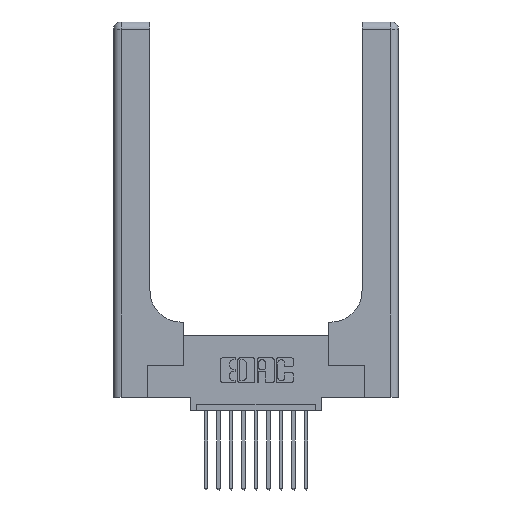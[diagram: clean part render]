
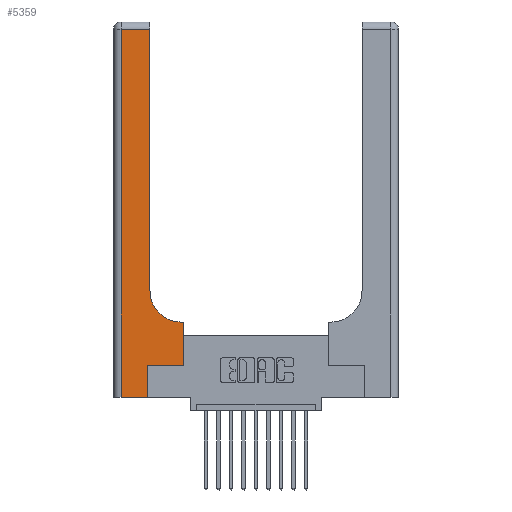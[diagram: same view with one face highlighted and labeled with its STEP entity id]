
A CAD part, top view. The second image highlights one B-rep face of the part: STEP entity #5359.
In plain terms, the highlighted planar face has unit normal (0, 0, 1).
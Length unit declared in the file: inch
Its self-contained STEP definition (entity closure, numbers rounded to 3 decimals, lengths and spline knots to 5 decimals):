
#34 = CARTESIAN_POINT ( 'NONE',  ( 0.2915, 0.6, 0.37 ) ) ;
#67 = EDGE_CURVE ( 'NONE', #10072, #5061, #8543, .T. ) ;
#112 = CARTESIAN_POINT ( 'NONE',  ( 0.5585, 0.25, 0.37 ) ) ;
#182 = ORIENTED_EDGE ( 'NONE', *, *, #4690, .T. ) ;
#774 = VERTEX_POINT ( 'NONE', #4327 ) ;
#806 = CARTESIAN_POINT ( 'NONE',  ( 0.2915, 3., 0.37 ) ) ;
#816 = CARTESIAN_POINT ( 'NONE',  ( 0.5415, 0.85, 0.37 ) ) ;
#1166 = CARTESIAN_POINT ( 'NONE',  ( 0.06, 2.94, 0.37 ) ) ;
#1419 = CARTESIAN_POINT ( 'NONE',  ( 0.269, 0.25, 0.37 ) ) ;
#1625 = EDGE_LOOP ( 'NONE', ( #16168, #10044, #14314, #6061, #182, #9993, #2555, #4718, #5748 ) ) ;
#1907 = AXIS2_PLACEMENT_3D ( 'NONE', #7122, #12544, #11205 ) ;
#2036 = DIRECTION ( 'NONE',  ( 1., 0., 0. ) ) ;
#2192 = VECTOR ( 'NONE', #16117, 39.37008 ) ;
#2379 = LINE ( 'NONE', #13437, #4820 ) ;
#2392 = LINE ( 'NONE', #16055, #7996 ) ;
#2555 = ORIENTED_EDGE ( 'NONE', *, *, #5330, .T. ) ;
#2706 = LINE ( 'NONE', #4996, #12505 ) ;
#2727 = DIRECTION ( 'NONE',  ( -1., 0., 0. ) ) ;
#3348 = DIRECTION ( 'NONE',  ( 0., 1., 0. ) ) ;
#3488 = DIRECTION ( 'NONE',  ( 1., 0., 0. ) ) ;
#3876 = CARTESIAN_POINT ( 'NONE',  ( 0.06, 3., 0.37 ) ) ;
#4117 = CARTESIAN_POINT ( 'NONE',  ( 0.269, 0., 0.37 ) ) ;
#4118 = CARTESIAN_POINT ( 'NONE',  ( 0.5415, 0.6, 0.37 ) ) ;
#4327 = CARTESIAN_POINT ( 'NONE',  ( 0.5585, 0.6, 0.37 ) ) ;
#4550 = AXIS2_PLACEMENT_3D ( 'NONE', #816, #9803, #3488 ) ;
#4690 = EDGE_CURVE ( 'NONE', #7204, #10072, #6435, .T. ) ;
#4718 = ORIENTED_EDGE ( 'NONE', *, *, #11504, .T. ) ;
#4820 = VECTOR ( 'NONE', #2036, 39.37008 ) ;
#4972 = LINE ( 'NONE', #3876, #14729 ) ;
#4996 = CARTESIAN_POINT ( 'NONE',  ( 0., 2.94, 0.37 ) ) ;
#5061 = VERTEX_POINT ( 'NONE', #112 ) ;
#5330 = EDGE_CURVE ( 'NONE', #5061, #774, #2392, .T. ) ;
#5359 = ADVANCED_FACE ( 'NONE', ( #16391 ), #13480, .F. ) ;
#5748 = ORIENTED_EDGE ( 'NONE', *, *, #10424, .T. ) ;
#6056 = DIRECTION ( 'NONE',  ( 1., 0., 0. ) ) ;
#6061 = ORIENTED_EDGE ( 'NONE', *, *, #14273, .T. ) ;
#6435 = LINE ( 'NONE', #4117, #12404 ) ;
#6474 = DIRECTION ( 'NONE',  ( -1., 0., 0. ) ) ;
#6517 = CIRCLE ( 'NONE', #4550, 0.25 ) ;
#6578 = CARTESIAN_POINT ( 'NONE',  ( 0.269, 0.25, 0.37 ) ) ;
#7122 = CARTESIAN_POINT ( 'NONE',  ( 0., 3., 0.37 ) ) ;
#7204 = VERTEX_POINT ( 'NONE', #14443 ) ;
#7996 = VECTOR ( 'NONE', #3348, 39.37008 ) ;
#8191 = LINE ( 'NONE', #806, #2192 ) ;
#8480 = VERTEX_POINT ( 'NONE', #12617 ) ;
#8543 = LINE ( 'NONE', #6578, #14733 ) ;
#8684 = CARTESIAN_POINT ( 'NONE',  ( 0.06, 0., 0.37 ) ) ;
#9544 = VERTEX_POINT ( 'NONE', #12246 ) ;
#9803 = DIRECTION ( 'NONE',  ( 0., 0., -1. ) ) ;
#9993 = ORIENTED_EDGE ( 'NONE', *, *, #67, .T. ) ;
#10044 = ORIENTED_EDGE ( 'NONE', *, *, #11347, .T. ) ;
#10072 = VERTEX_POINT ( 'NONE', #1419 ) ;
#10278 = DIRECTION ( 'NONE',  ( 0., -1., 0. ) ) ;
#10424 = EDGE_CURVE ( 'NONE', #15781, #8480, #6517, .T. ) ;
#11205 = DIRECTION ( 'NONE',  ( -1., 0., 0. ) ) ;
#11347 = EDGE_CURVE ( 'NONE', #9544, #14542, #2706, .T. ) ;
#11461 = VERTEX_POINT ( 'NONE', #8684 ) ;
#11504 = EDGE_CURVE ( 'NONE', #774, #15781, #13903, .T. ) ;
#12246 = CARTESIAN_POINT ( 'NONE',  ( 0.2915, 2.94, 0.37 ) ) ;
#12404 = VECTOR ( 'NONE', #13872, 39.37008 ) ;
#12505 = VECTOR ( 'NONE', #2727, 39.37008 ) ;
#12544 = DIRECTION ( 'NONE',  ( 0., 0., -1. ) ) ;
#12617 = CARTESIAN_POINT ( 'NONE',  ( 0.2915, 0.85, 0.37 ) ) ;
#13437 = CARTESIAN_POINT ( 'NONE',  ( 0., 0., 0.37 ) ) ;
#13480 = PLANE ( 'NONE',  #1907 ) ;
#13872 = DIRECTION ( 'NONE',  ( 0., 1., 0. ) ) ;
#13903 = LINE ( 'NONE', #34, #14479 ) ;
#14273 = EDGE_CURVE ( 'NONE', #11461, #7204, #2379, .T. ) ;
#14314 = ORIENTED_EDGE ( 'NONE', *, *, #15565, .T. ) ;
#14325 = EDGE_CURVE ( 'NONE', #8480, #9544, #8191, .T. ) ;
#14443 = CARTESIAN_POINT ( 'NONE',  ( 0.269, 0., 0.37 ) ) ;
#14479 = VECTOR ( 'NONE', #6474, 39.37008 ) ;
#14542 = VERTEX_POINT ( 'NONE', #1166 ) ;
#14729 = VECTOR ( 'NONE', #10278, 39.37008 ) ;
#14733 = VECTOR ( 'NONE', #6056, 39.37008 ) ;
#15565 = EDGE_CURVE ( 'NONE', #14542, #11461, #4972, .T. ) ;
#15781 = VERTEX_POINT ( 'NONE', #4118 ) ;
#16055 = CARTESIAN_POINT ( 'NONE',  ( 0.5585, 0.25, 0.37 ) ) ;
#16117 = DIRECTION ( 'NONE',  ( 0., 1., 0. ) ) ;
#16168 = ORIENTED_EDGE ( 'NONE', *, *, #14325, .T. ) ;
#16391 = FACE_OUTER_BOUND ( 'NONE', #1625, .T. ) ;
